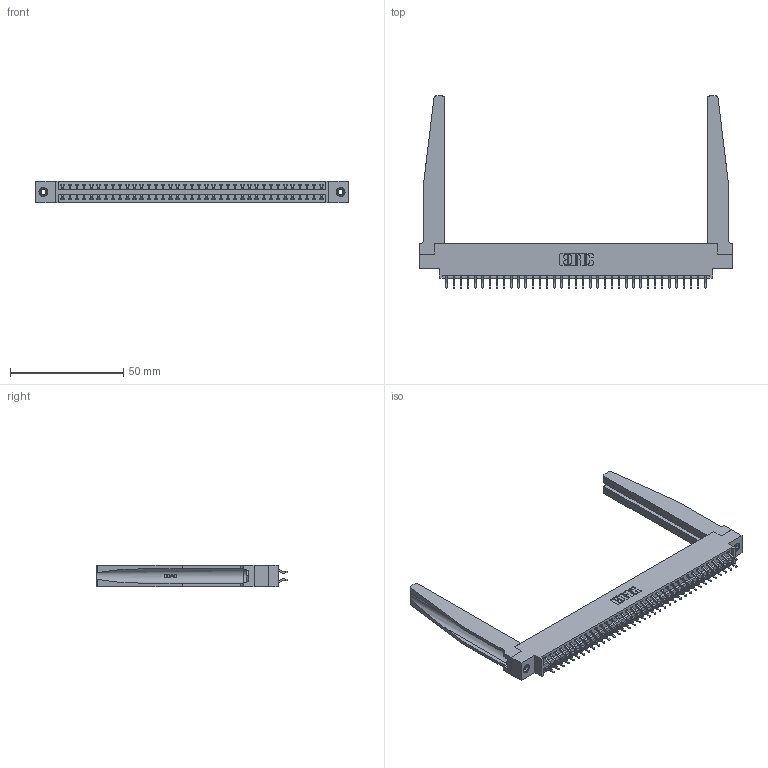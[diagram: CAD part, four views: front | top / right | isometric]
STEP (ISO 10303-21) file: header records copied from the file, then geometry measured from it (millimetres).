
FILE_DESCRIPTION (( 'STEP AP203' ), '1' );
FILE_NAME ('396-074-556-878.STEP', '2019-11-02T12:47:01', ( '' ), ( '' ), 'SwSTEP 2.0', 'SolidWorks 2016', '' );
FILE_SCHEMA (( 'CONFIG_CONTROL_DESIGN' ));
Length unit declared in the file: inch
Products named in the file (5): 345-250-001_345-250-001-102; 396-074-556-878; 346 Part_0.170 Offset - 0.156 Dia-TH; 345-292-001_556 Tail; 346-220-078_345-220-078
Assembly tree (79 placements, depth 2):
  396-074-556-878
    346 Part_0.170 Offset - 0.156 Dia-TH
    345-292-001_556 Tail  x74
    346-220-078_345-220-078  x2
    345-250-001_345-250-001-102  x2
Bounding box: 138.05 x 84.84 x 9.4 mm (x, y, z)
Volume: 20174 mm3; surface area: 24803.6 mm2
Topology: 79 solids, 79 shells, 4652 faces, 13751 edges, 9058 vertices
Faces by surface type: plane 3108, cylinder 1492, bspline 36, cone 12, torus 4
Entity records: 29920 total; most frequent: CARTESIAN_POINT 5891, ORIENTED_EDGE 4702, DIRECTION 4217, EDGE_CURVE 2351, LINE 1969, VECTOR 1969, VERTEX_POINT 1560, AXIS2_PLACEMENT_3D 1124
